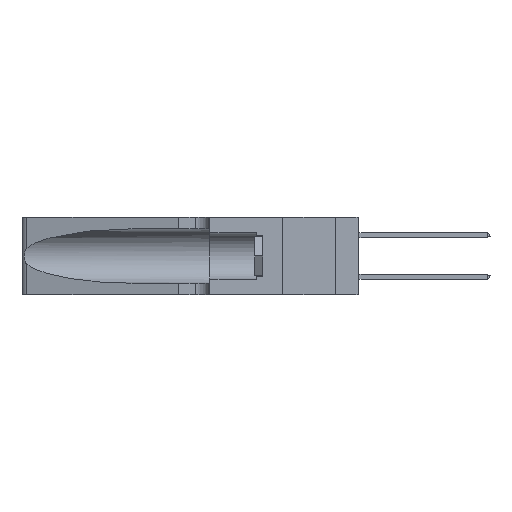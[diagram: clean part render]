
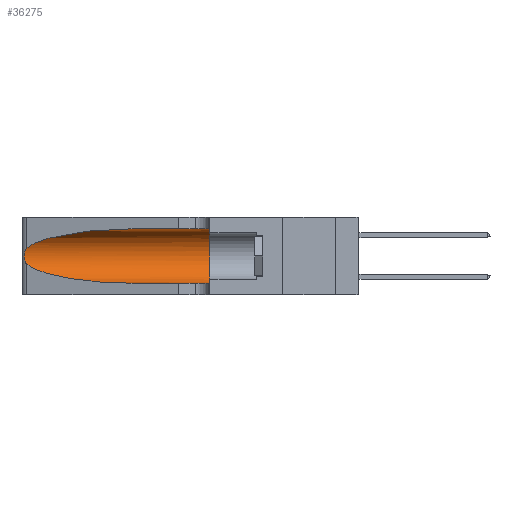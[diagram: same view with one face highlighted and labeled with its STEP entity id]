
A CAD part, left-side view. The second image highlights one B-rep face of the part: STEP entity #36275.
In plain terms, the highlighted cylindrical face has radius 3.308 mm (diameter 6.617 mm), a partial arc.
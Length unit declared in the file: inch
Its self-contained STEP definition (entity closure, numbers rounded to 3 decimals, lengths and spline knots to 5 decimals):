
#1544 = VERTEX_POINT ( 'NONE', #31546 ) ;
#1914 = VERTEX_POINT ( 'NONE', #20712 ) ;
#1935 = CARTESIAN_POINT ( 'NONE',  ( 0.25487, 1.22718, 0.14631 ) ) ;
#2062 = CARTESIAN_POINT ( 'NONE',  ( 0.18966, 0.96281, 0.05475 ) ) ;
#2522 = DIRECTION ( 'NONE',  ( 0., -1., 0. ) ) ;
#3919 = EDGE_CURVE ( 'NONE', #1914, #24307, #9391, .T. ) ;
#4087 = ORIENTED_EDGE ( 'NONE', *, *, #6066, .T. ) ;
#4908 = CARTESIAN_POINT ( 'NONE',  ( 0.25639, 1.23184, 0.21858 ) ) ;
#5735 = CARTESIAN_POINT ( 'NONE',  ( 0.1305, 1.61858, 0.185 ) ) ;
#5770 = AXIS2_PLACEMENT_3D ( 'NONE', #11503, #33140, #14630 ) ;
#5855 = CARTESIAN_POINT ( 'NONE',  ( 0.18966, 0.96281, 0.31525 ) ) ;
#6066 = EDGE_CURVE ( 'NONE', #23477, #1544, #11381, .T. ) ;
#6102 = LINE ( 'NONE', #9936, #21564 ) ;
#7230 = AXIS2_PLACEMENT_3D ( 'NONE', #5735, #2522, #21135 ) ;
#7377 = CIRCLE ( 'NONE', #5770, 0.13025 ) ;
#7656 = EDGE_LOOP ( 'NONE', ( #22471, #26081, #22473, #4087, #9787, #10150 ) ) ;
#7725 = FACE_OUTER_BOUND ( 'NONE', #7656, .T. ) ;
#8002 = CARTESIAN_POINT ( 'NONE',  ( 0.25854, 1.2359, 0.20912 ) ) ;
#8809 = CARTESIAN_POINT ( 'NONE',  ( 0.1305, 0.72297, 0.31525 ) ) ;
#9355 = VERTEX_POINT ( 'NONE', #25744 ) ;
#9391 =( BOUNDED_CURVE ( )  B_SPLINE_CURVE ( 3, ( #8809, #5855, #30594, #12042 ),
 .UNSPECIFIED., .F., .T. ) 
 B_SPLINE_CURVE_WITH_KNOTS ( ( 4, 4 ),
 ( 1.5708, 2.84003 ),
 .UNSPECIFIED. ) 
 CURVE ( )  GEOMETRIC_REPRESENTATION_ITEM ( )  RATIONAL_B_SPLINE_CURVE ( ( 1., 0.87, 0.87, 1. ) ) 
 REPRESENTATION_ITEM ( '' )  );
#9787 = ORIENTED_EDGE ( 'NONE', *, *, #23749, .F. ) ;
#9936 = CARTESIAN_POINT ( 'NONE',  ( 0.1305, 1.61858, 0.31525 ) ) ;
#10150 = ORIENTED_EDGE ( 'NONE', *, *, #29364, .F. ) ;
#10483 = B_SPLINE_CURVE_WITH_KNOTS ( 'NONE', 3,
 ( #17175, #20286, #4908, #26512, #8002, #29602, #11072, #32705, #14203, #35736, #17304, #38796, #20425, #1935 ),
 .UNSPECIFIED., .F., .F.,
 ( 4, 2, 2, 2, 2, 2, 4 ),
 ( 0., 0.00027, 0.00053, 0.00107, 0.0016, 0.00187, 0.00214 ),
 .UNSPECIFIED. ) ;
#11072 = CARTESIAN_POINT ( 'NONE',  ( 0.26075, 1.23896, 0.19203 ) ) ;
#11381 = LINE ( 'NONE', #13477, #35033 ) ;
#11503 = CARTESIAN_POINT ( 'NONE',  ( 0.1305, 0.35, 0.185 ) ) ;
#12042 = CARTESIAN_POINT ( 'NONE',  ( 0.25487, 1.22718, 0.22369 ) ) ;
#13064 = DIRECTION ( 'NONE',  ( 0., -1., 0. ) ) ;
#13477 = CARTESIAN_POINT ( 'NONE',  ( 0.1305, 1.61858, 0.05475 ) ) ;
#14203 = CARTESIAN_POINT ( 'NONE',  ( 0.26017, 1.23833, 0.17102 ) ) ;
#14320 = CARTESIAN_POINT ( 'NONE',  ( 0.2373, 1.15595, 0.08982 ) ) ;
#14630 = DIRECTION ( 'NONE',  ( 0., 0., 1. ) ) ;
#14953 = CYLINDRICAL_SURFACE ( 'NONE', #7230, 0.13025 ) ;
#15693 = EDGE_CURVE ( 'NONE', #24307, #25238, #10483, .T. ) ;
#17175 = CARTESIAN_POINT ( 'NONE',  ( 0.25487, 1.22718, 0.22369 ) ) ;
#17304 = CARTESIAN_POINT ( 'NONE',  ( 0.25789, 1.23486, 0.15765 ) ) ;
#20286 = CARTESIAN_POINT ( 'NONE',  ( 0.25555, 1.22994, 0.2215 ) ) ;
#20425 = CARTESIAN_POINT ( 'NONE',  ( 0.25555, 1.22993, 0.14849 ) ) ;
#20712 = CARTESIAN_POINT ( 'NONE',  ( 0.1305, 0.72297, 0.31525 ) ) ;
#21135 = DIRECTION ( 'NONE',  ( 0., 0., -1. ) ) ;
#21157 = CARTESIAN_POINT ( 'NONE',  ( 0.25487, 1.22718, 0.14631 ) ) ;
#21564 = VECTOR ( 'NONE', #13064, 39.37008 ) ;
#22471 = ORIENTED_EDGE ( 'NONE', *, *, #3919, .T. ) ;
#22473 = ORIENTED_EDGE ( 'NONE', *, *, #24352, .T. ) ;
#23477 = VERTEX_POINT ( 'NONE', #25896 ) ;
#23527 = CARTESIAN_POINT ( 'NONE',  ( 0.25487, 1.22718, 0.14631 ) ) ;
#23649 = CARTESIAN_POINT ( 'NONE',  ( 0.1305, 0.72297, 0.05475 ) ) ;
#23749 = EDGE_CURVE ( 'NONE', #9355, #1544, #7377, .T. ) ;
#24307 = VERTEX_POINT ( 'NONE', #29587 ) ;
#24352 = EDGE_CURVE ( 'NONE', #25238, #23477, #38244, .T. ) ;
#25238 = VERTEX_POINT ( 'NONE', #21157 ) ;
#25744 = CARTESIAN_POINT ( 'NONE',  ( 0.1305, 0.35, 0.31525 ) ) ;
#25896 = CARTESIAN_POINT ( 'NONE',  ( 0.1305, 0.72297, 0.05475 ) ) ;
#26081 = ORIENTED_EDGE ( 'NONE', *, *, #15693, .T. ) ;
#26512 = CARTESIAN_POINT ( 'NONE',  ( 0.25787, 1.23484, 0.2124 ) ) ;
#29364 = EDGE_CURVE ( 'NONE', #1914, #9355, #6102, .T. ) ;
#29587 = CARTESIAN_POINT ( 'NONE',  ( 0.25487, 1.22718, 0.22369 ) ) ;
#29602 = CARTESIAN_POINT ( 'NONE',  ( 0.26018, 1.23835, 0.19895 ) ) ;
#30594 = CARTESIAN_POINT ( 'NONE',  ( 0.2373, 1.15595, 0.28018 ) ) ;
#31546 = CARTESIAN_POINT ( 'NONE',  ( 0.1305, 0.35, 0.05475 ) ) ;
#32004 = DIRECTION ( 'NONE',  ( 0., -1., 0. ) ) ;
#32705 = CARTESIAN_POINT ( 'NONE',  ( 0.26075, 1.23896, 0.178 ) ) ;
#33140 = DIRECTION ( 'NONE',  ( 0., 1., 0. ) ) ;
#35033 = VECTOR ( 'NONE', #32004, 39.37008 ) ;
#35736 = CARTESIAN_POINT ( 'NONE',  ( 0.25856, 1.23593, 0.16098 ) ) ;
#36275 = ADVANCED_FACE ( 'NONE', ( #7725 ), #14953, .F. ) ;
#38244 =( BOUNDED_CURVE ( )  B_SPLINE_CURVE ( 3, ( #23527, #14320, #2062, #23649 ),
 .UNSPECIFIED., .F., .T. ) 
 B_SPLINE_CURVE_WITH_KNOTS ( ( 4, 4 ),
 ( 3.44316, 4.71239 ),
 .UNSPECIFIED. ) 
 CURVE ( )  GEOMETRIC_REPRESENTATION_ITEM ( )  RATIONAL_B_SPLINE_CURVE ( ( 1., 0.87, 0.87, 1. ) ) 
 REPRESENTATION_ITEM ( '' )  );
#38796 = CARTESIAN_POINT ( 'NONE',  ( 0.25639, 1.23186, 0.15144 ) ) ;
